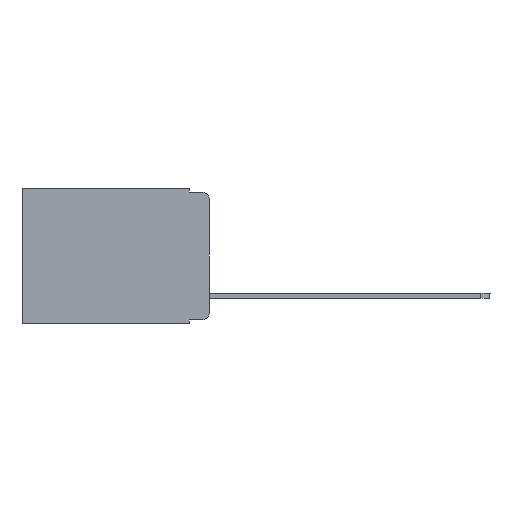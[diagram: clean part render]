
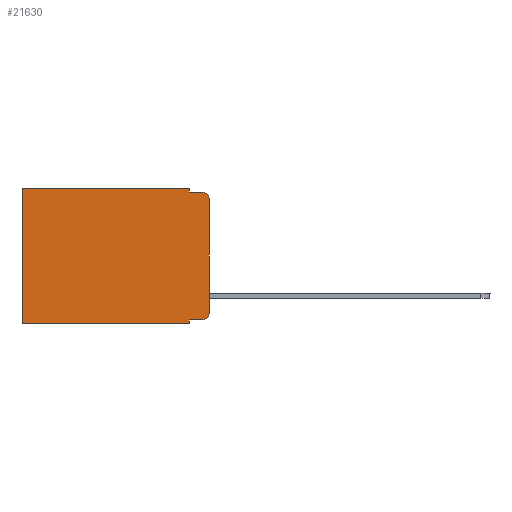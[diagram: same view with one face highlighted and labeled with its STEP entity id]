
A CAD part, left-side view. The second image highlights one B-rep face of the part: STEP entity #21630.
In plain terms, the highlighted planar face has unit normal (-1, 0, 0).
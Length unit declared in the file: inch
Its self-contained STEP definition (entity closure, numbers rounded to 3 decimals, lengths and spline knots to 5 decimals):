
#153 = CARTESIAN_POINT ( 'NONE',  ( 0.298, 0.051, -0.01 ) ) ;
#870 = CARTESIAN_POINT ( 'NONE',  ( 0.298, 0.051, -0.343 ) ) ;
#1385 = VERTEX_POINT ( 'NONE', #17492 ) ;
#1773 = CARTESIAN_POINT ( 'NONE',  ( 0.298, 0.02, -0.03 ) ) ;
#2555 = EDGE_CURVE ( 'NONE', #21903, #5062, #3505, .T. ) ;
#2571 = ORIENTED_EDGE ( 'NONE', *, *, #9074, .F. ) ;
#2584 = CARTESIAN_POINT ( 'NONE',  ( 0.298, 0.051, -0.01 ) ) ;
#3429 = CARTESIAN_POINT ( 'NONE',  ( 0.298, 0., -0.03 ) ) ;
#3505 = LINE ( 'NONE', #4988, #20313 ) ;
#3569 = DIRECTION ( 'NONE',  ( 0., 1., 0. ) ) ;
#4046 = EDGE_CURVE ( 'NONE', #21903, #1385, #10634, .T. ) ;
#4435 = DIRECTION ( 'NONE',  ( 0., -1., 0. ) ) ;
#4835 = CARTESIAN_POINT ( 'NONE',  ( 0.298, 0.02, -0.313 ) ) ;
#4988 = CARTESIAN_POINT ( 'NONE',  ( 0.298, 0.051, 0. ) ) ;
#5062 = VERTEX_POINT ( 'NONE', #153 ) ;
#5097 = ORIENTED_EDGE ( 'NONE', *, *, #21891, .F. ) ;
#5106 = CIRCLE ( 'NONE', #11293, 0.02 ) ;
#5511 = CARTESIAN_POINT ( 'NONE',  ( 0.298, 0., -0.313 ) ) ;
#5538 = DIRECTION ( 'NONE',  ( 0., 0., -1. ) ) ;
#5961 = DIRECTION ( 'NONE',  ( 0., 0., -1. ) ) ;
#6062 = VECTOR ( 'NONE', #16311, 39.37008 ) ;
#6993 = CARTESIAN_POINT ( 'NONE',  ( 0.298, 0., -0.343 ) ) ;
#7335 = DIRECTION ( 'NONE',  ( 0., 1., 0. ) ) ;
#7374 = VERTEX_POINT ( 'NONE', #16602 ) ;
#7500 = ORIENTED_EDGE ( 'NONE', *, *, #2555, .F. ) ;
#7576 = VERTEX_POINT ( 'NONE', #21185 ) ;
#7905 = CARTESIAN_POINT ( 'NONE',  ( 0.298, 0.051, 0. ) ) ;
#8036 = VERTEX_POINT ( 'NONE', #3429 ) ;
#8223 = CARTESIAN_POINT ( 'NONE',  ( 0.298, 0., 0. ) ) ;
#8321 = LINE ( 'NONE', #20352, #9593 ) ;
#8452 = ORIENTED_EDGE ( 'NONE', *, *, #11115, .T. ) ;
#9074 = EDGE_CURVE ( 'NONE', #7374, #17753, #9378, .T. ) ;
#9239 = EDGE_CURVE ( 'NONE', #8036, #15716, #15257, .T. ) ;
#9378 = LINE ( 'NONE', #7905, #6062 ) ;
#9541 = CARTESIAN_POINT ( 'NONE',  ( 0.298, 0.051, 0. ) ) ;
#9593 = VECTOR ( 'NONE', #15575, 39.37008 ) ;
#9624 = DIRECTION ( 'NONE',  ( -1., 0., 0. ) ) ;
#10352 = ORIENTED_EDGE ( 'NONE', *, *, #19668, .F. ) ;
#10460 = DIRECTION ( 'NONE',  ( 0., 0., -1. ) ) ;
#10634 = LINE ( 'NONE', #22452, #20717 ) ;
#10831 = VECTOR ( 'NONE', #7335, 39.37008 ) ;
#11115 = EDGE_CURVE ( 'NONE', #8036, #17499, #21453, .T. ) ;
#11293 = AXIS2_PLACEMENT_3D ( 'NONE', #4835, #9624, #13471 ) ;
#12429 = LINE ( 'NONE', #6993, #10831 ) ;
#12913 = VECTOR ( 'NONE', #22188, 39.37008 ) ;
#12994 = FACE_OUTER_BOUND ( 'NONE', #21000, .T. ) ;
#13471 = DIRECTION ( 'NONE',  ( 0., 0., -1. ) ) ;
#13561 = EDGE_CURVE ( 'NONE', #1385, #7576, #8321, .T. ) ;
#13721 = DIRECTION ( 'NONE',  ( -1., 0., 0. ) ) ;
#14563 = AXIS2_PLACEMENT_3D ( 'NONE', #1773, #13721, #5538 ) ;
#14615 = ORIENTED_EDGE ( 'NONE', *, *, #22404, .T. ) ;
#15139 = DIRECTION ( 'NONE',  ( 1., 0., 0. ) ) ;
#15257 = LINE ( 'NONE', #18562, #12913 ) ;
#15575 = DIRECTION ( 'NONE',  ( 0., 0., -1. ) ) ;
#15716 = VERTEX_POINT ( 'NONE', #5511 ) ;
#15935 = ORIENTED_EDGE ( 'NONE', *, *, #4046, .T. ) ;
#16311 = DIRECTION ( 'NONE',  ( 0., 0., -1. ) ) ;
#16359 = DIRECTION ( 'NONE',  ( 0., -1., 0. ) ) ;
#16421 = PLANE ( 'NONE',  #17429 ) ;
#16602 = CARTESIAN_POINT ( 'NONE',  ( 0.298, 0.051, -0.333 ) ) ;
#17429 = AXIS2_PLACEMENT_3D ( 'NONE', #8223, #15139, #5961 ) ;
#17492 = CARTESIAN_POINT ( 'NONE',  ( 0.298, 0.473, 0. ) ) ;
#17499 = VERTEX_POINT ( 'NONE', #20681 ) ;
#17753 = VERTEX_POINT ( 'NONE', #870 ) ;
#17801 = ORIENTED_EDGE ( 'NONE', *, *, #9239, .F. ) ;
#18030 = VERTEX_POINT ( 'NONE', #19156 ) ;
#18169 = LINE ( 'NONE', #2584, #22157 ) ;
#18262 = ORIENTED_EDGE ( 'NONE', *, *, #19357, .T. ) ;
#18430 = VECTOR ( 'NONE', #16359, 39.37008 ) ;
#18562 = CARTESIAN_POINT ( 'NONE',  ( 0.298, 0., 0. ) ) ;
#19156 = CARTESIAN_POINT ( 'NONE',  ( 0.298, 0.02, -0.333 ) ) ;
#19357 = EDGE_CURVE ( 'NONE', #7374, #18030, #19518, .T. ) ;
#19518 = LINE ( 'NONE', #19742, #18430 ) ;
#19668 = EDGE_CURVE ( 'NONE', #17753, #7576, #12429, .T. ) ;
#19742 = CARTESIAN_POINT ( 'NONE',  ( 0.298, 0.051, -0.333 ) ) ;
#20313 = VECTOR ( 'NONE', #10460, 39.37008 ) ;
#20352 = CARTESIAN_POINT ( 'NONE',  ( 0.298, 0.473, 0. ) ) ;
#20681 = CARTESIAN_POINT ( 'NONE',  ( 0.298, 0.02, -0.01 ) ) ;
#20717 = VECTOR ( 'NONE', #3569, 39.37008 ) ;
#21000 = EDGE_LOOP ( 'NONE', ( #17801, #8452, #5097, #7500, #15935, #22461, #10352, #2571, #18262, #14615 ) ) ;
#21185 = CARTESIAN_POINT ( 'NONE',  ( 0.298, 0.473, -0.343 ) ) ;
#21453 = CIRCLE ( 'NONE', #14563, 0.02 ) ;
#21630 = ADVANCED_FACE ( 'NONE', ( #12994 ), #16421, .F. ) ;
#21891 = EDGE_CURVE ( 'NONE', #5062, #17499, #18169, .T. ) ;
#21903 = VERTEX_POINT ( 'NONE', #9541 ) ;
#22157 = VECTOR ( 'NONE', #4435, 39.37008 ) ;
#22188 = DIRECTION ( 'NONE',  ( 0., 0., -1. ) ) ;
#22404 = EDGE_CURVE ( 'NONE', #18030, #15716, #5106, .T. ) ;
#22452 = CARTESIAN_POINT ( 'NONE',  ( 0.298, 0., 0. ) ) ;
#22461 = ORIENTED_EDGE ( 'NONE', *, *, #13561, .T. ) ;
